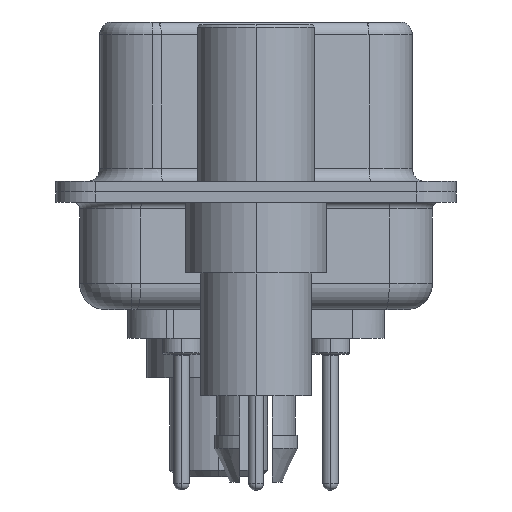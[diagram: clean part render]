
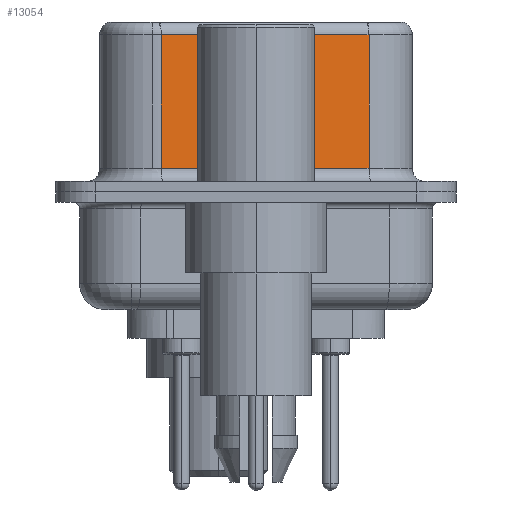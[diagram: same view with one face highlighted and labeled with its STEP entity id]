
A CAD part, left-side view. The second image highlights one B-rep face of the part: STEP entity #13054.
In plain terms, the highlighted planar face has unit normal (-0.985, -0.174, 0).
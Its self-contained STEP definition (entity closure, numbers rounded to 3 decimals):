
#640 = LINE ( 'NONE', #16646, #26119 ) ;
#1454 = DIRECTION ( 'NONE',  ( -0.174, 0.985, 0. ) ) ;
#2463 = EDGE_CURVE ( 'NONE', #12001, #21470, #640, .T. ) ;
#3151 = CARTESIAN_POINT ( 'NONE',  ( 5.132, -4.322, 6.02 ) ) ;
#6660 = ORIENTED_EDGE ( 'NONE', *, *, #27952, .T. ) ;
#6706 = LINE ( 'NONE', #29796, #7519 ) ;
#7262 = LINE ( 'NONE', #15519, #12345 ) ;
#7519 = VECTOR ( 'NONE', #19518, 1000. ) ;
#8909 = EDGE_LOOP ( 'NONE', ( #14513, #22676, #6660, #22934 ) ) ;
#9380 = VECTOR ( 'NONE', #32273, 1000. ) ;
#12001 = VERTEX_POINT ( 'NONE', #3151 ) ;
#12345 = VECTOR ( 'NONE', #22981, 1000. ) ;
#12840 = CARTESIAN_POINT ( 'NONE',  ( 3.73, 3.628, 0.9 ) ) ;
#13054 = ADVANCED_FACE ( 'NONE', ( #31426 ), #29357, .F. ) ;
#13838 = EDGE_CURVE ( 'NONE', #12001, #15850, #7262, .T. ) ;
#14513 = ORIENTED_EDGE ( 'NONE', *, *, #2463, .F. ) ;
#15519 = CARTESIAN_POINT ( 'NONE',  ( 5.132, -4.322, 6.02 ) ) ;
#15850 = VERTEX_POINT ( 'NONE', #23977 ) ;
#16017 = LINE ( 'NONE', #19562, #9380 ) ;
#16097 = EDGE_CURVE ( 'NONE', #16266, #21470, #6706, .T. ) ;
#16266 = VERTEX_POINT ( 'NONE', #12840 ) ;
#16646 = CARTESIAN_POINT ( 'NONE',  ( 5.132, -4.322, 6.52 ) ) ;
#16679 = DIRECTION ( 'NONE',  ( 0.985, 0.174, 0. ) ) ;
#17103 = AXIS2_PLACEMENT_3D ( 'NONE', #19068, #16679, #1454 ) ;
#18682 = DIRECTION ( 'NONE',  ( 0., 0., -1. ) ) ;
#19068 = CARTESIAN_POINT ( 'NONE',  ( 5.132, -4.322, 6.52 ) ) ;
#19518 = DIRECTION ( 'NONE',  ( 0.174, -0.985, 0. ) ) ;
#19562 = CARTESIAN_POINT ( 'NONE',  ( 3.73, 3.628, 6.52 ) ) ;
#21470 = VERTEX_POINT ( 'NONE', #30335 ) ;
#22676 = ORIENTED_EDGE ( 'NONE', *, *, #13838, .T. ) ;
#22934 = ORIENTED_EDGE ( 'NONE', *, *, #16097, .T. ) ;
#22981 = DIRECTION ( 'NONE',  ( -0.174, 0.985, 0. ) ) ;
#23977 = CARTESIAN_POINT ( 'NONE',  ( 3.73, 3.628, 6.02 ) ) ;
#26119 = VECTOR ( 'NONE', #18682, 1000. ) ;
#27952 = EDGE_CURVE ( 'NONE', #15850, #16266, #16017, .T. ) ;
#29357 = PLANE ( 'NONE',  #17103 ) ;
#29796 = CARTESIAN_POINT ( 'NONE',  ( 5.132, -4.322, 0.9 ) ) ;
#30335 = CARTESIAN_POINT ( 'NONE',  ( 5.132, -4.322, 0.9 ) ) ;
#31426 = FACE_OUTER_BOUND ( 'NONE', #8909, .T. ) ;
#32273 = DIRECTION ( 'NONE',  ( 0., 0., -1. ) ) ;
